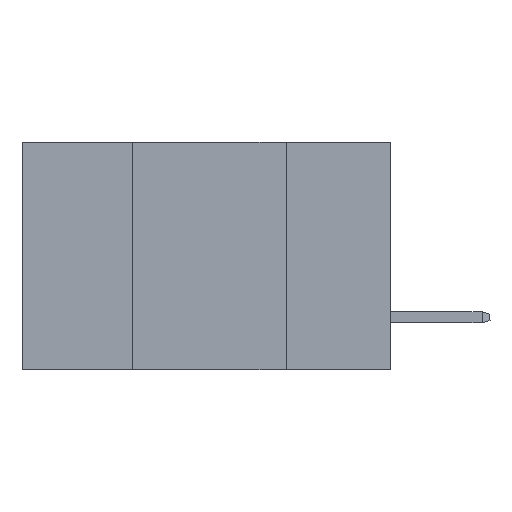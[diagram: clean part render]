
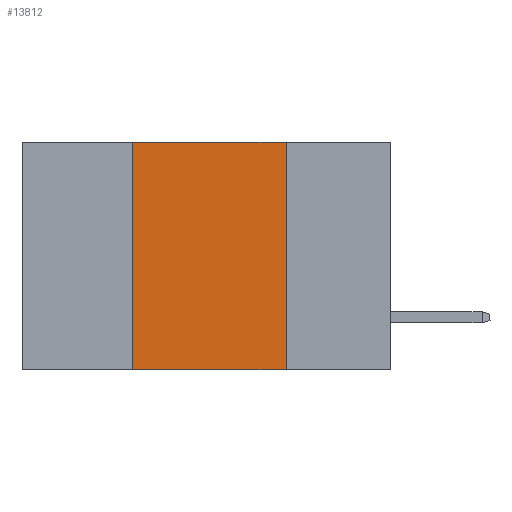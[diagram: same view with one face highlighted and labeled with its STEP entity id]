
A CAD part, left-side view. The second image highlights one B-rep face of the part: STEP entity #13812.
In plain terms, the highlighted planar face has unit normal (-1, 0, 0).
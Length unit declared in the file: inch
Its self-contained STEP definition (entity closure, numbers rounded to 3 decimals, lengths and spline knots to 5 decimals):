
#9 = DIRECTION ( 'NONE',  ( 1., 0., 0. ) ) ;
#76 = EDGE_CURVE ( 'NONE', #7418, #11027, #13836, .T. ) ;
#334 = VECTOR ( 'NONE', #441, 39.37008 ) ;
#441 = DIRECTION ( 'NONE',  ( 0., -1., 0. ) ) ;
#813 = VECTOR ( 'NONE', #13201, 39.37008 ) ;
#927 = CARTESIAN_POINT ( 'NONE',  ( 0., 0.6, -0.37 ) ) ;
#1331 = FACE_OUTER_BOUND ( 'NONE', #3844, .T. ) ;
#1534 = CARTESIAN_POINT ( 'NONE',  ( 0., 0.6, 0. ) ) ;
#3844 = EDGE_LOOP ( 'NONE', ( #9374, #9297, #16349, #10574 ) ) ;
#4609 = CARTESIAN_POINT ( 'NONE',  ( 0., 0.42, 0. ) ) ;
#4781 = EDGE_CURVE ( 'NONE', #7418, #15670, #11226, .T. ) ;
#4955 = DIRECTION ( 'NONE',  ( 0., -1., 0. ) ) ;
#5079 = AXIS2_PLACEMENT_3D ( 'NONE', #8688, #9, #11987 ) ;
#5247 = PLANE ( 'NONE',  #5079 ) ;
#6614 = CARTESIAN_POINT ( 'NONE',  ( 0., 0.42, -0.37 ) ) ;
#7165 = CARTESIAN_POINT ( 'NONE',  ( 0., 0.17, 0. ) ) ;
#7418 = VERTEX_POINT ( 'NONE', #6614 ) ;
#8688 = CARTESIAN_POINT ( 'NONE',  ( 0., 0.6, 0. ) ) ;
#9297 = ORIENTED_EDGE ( 'NONE', *, *, #17045, .F. ) ;
#9374 = ORIENTED_EDGE ( 'NONE', *, *, #13044, .F. ) ;
#10574 = ORIENTED_EDGE ( 'NONE', *, *, #76, .T. ) ;
#11027 = VERTEX_POINT ( 'NONE', #12659 ) ;
#11226 = LINE ( 'NONE', #4609, #15401 ) ;
#11591 = CARTESIAN_POINT ( 'NONE',  ( 0., 0.17, 0. ) ) ;
#11987 = DIRECTION ( 'NONE',  ( 0., 0., -1. ) ) ;
#12659 = CARTESIAN_POINT ( 'NONE',  ( 0., 0.17, -0.37 ) ) ;
#13044 = EDGE_CURVE ( 'NONE', #16584, #11027, #13757, .T. ) ;
#13201 = DIRECTION ( 'NONE',  ( 0., 0., -1. ) ) ;
#13757 = LINE ( 'NONE', #11591, #813 ) ;
#13812 = ADVANCED_FACE ( 'NONE', ( #1331 ), #5247, .F. ) ;
#13825 = VECTOR ( 'NONE', #4955, 39.37008 ) ;
#13836 = LINE ( 'NONE', #927, #334 ) ;
#14320 = LINE ( 'NONE', #1534, #13825 ) ;
#15401 = VECTOR ( 'NONE', #19249, 39.37008 ) ;
#15670 = VERTEX_POINT ( 'NONE', #19192 ) ;
#16349 = ORIENTED_EDGE ( 'NONE', *, *, #4781, .F. ) ;
#16584 = VERTEX_POINT ( 'NONE', #7165 ) ;
#17045 = EDGE_CURVE ( 'NONE', #15670, #16584, #14320, .T. ) ;
#19192 = CARTESIAN_POINT ( 'NONE',  ( 0., 0.42, 0. ) ) ;
#19249 = DIRECTION ( 'NONE',  ( 0., 0., 1. ) ) ;
